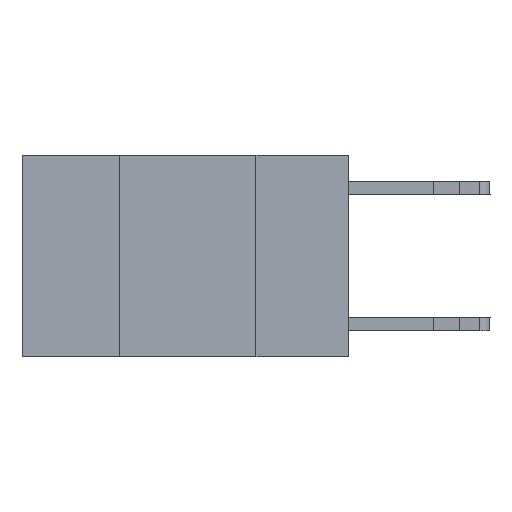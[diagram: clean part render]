
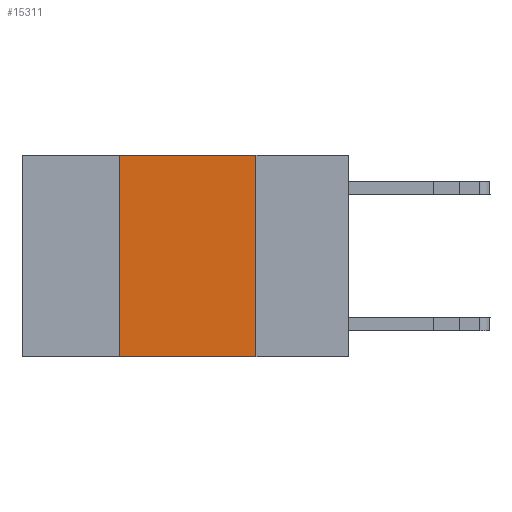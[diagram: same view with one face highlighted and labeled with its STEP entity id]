
A CAD part, left-side view. The second image highlights one B-rep face of the part: STEP entity #15311.
In plain terms, the highlighted planar face has unit normal (-1, 0, 0).
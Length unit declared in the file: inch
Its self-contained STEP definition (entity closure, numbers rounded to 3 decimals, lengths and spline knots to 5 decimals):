
#153 = PLANE ( 'NONE',  #7304 ) ;
#226 = DIRECTION ( 'NONE',  ( 0., -1., 0. ) ) ;
#289 = VERTEX_POINT ( 'NONE', #11946 ) ;
#1091 = EDGE_CURVE ( 'NONE', #289, #7516, #4039, .T. ) ;
#1394 = CARTESIAN_POINT ( 'NONE',  ( 0., 0.6, 0. ) ) ;
#1438 = VERTEX_POINT ( 'NONE', #4000 ) ;
#1507 = CARTESIAN_POINT ( 'NONE',  ( 0., 0.6, -0.37 ) ) ;
#2145 = EDGE_CURVE ( 'NONE', #1438, #4089, #7853, .T. ) ;
#2766 = ORIENTED_EDGE ( 'NONE', *, *, #5852, .F. ) ;
#3180 = VECTOR ( 'NONE', #7552, 39.37008 ) ;
#3196 = EDGE_CURVE ( 'NONE', #1438, #289, #8893, .T. ) ;
#3746 = DIRECTION ( 'NONE',  ( 0., 0., -1. ) ) ;
#4000 = CARTESIAN_POINT ( 'NONE',  ( 0., 0.42, -0.37 ) ) ;
#4039 = LINE ( 'NONE', #1394, #7570 ) ;
#4089 = VERTEX_POINT ( 'NONE', #15460 ) ;
#4158 = ORIENTED_EDGE ( 'NONE', *, *, #1091, .F. ) ;
#4558 = EDGE_LOOP ( 'NONE', ( #2766, #4158, #15081, #15997 ) ) ;
#4674 = DIRECTION ( 'NONE',  ( 0., 0., -1. ) ) ;
#4994 = LINE ( 'NONE', #15204, #8172 ) ;
#5852 = EDGE_CURVE ( 'NONE', #7516, #4089, #4994, .T. ) ;
#5996 = CARTESIAN_POINT ( 'NONE',  ( 0., 0.17, 0. ) ) ;
#6511 = CARTESIAN_POINT ( 'NONE',  ( 0., 0.6, 0. ) ) ;
#7304 = AXIS2_PLACEMENT_3D ( 'NONE', #6511, #15384, #4674 ) ;
#7516 = VERTEX_POINT ( 'NONE', #5996 ) ;
#7552 = DIRECTION ( 'NONE',  ( 0., 0., 1. ) ) ;
#7570 = VECTOR ( 'NONE', #11741, 39.37008 ) ;
#7853 = LINE ( 'NONE', #1507, #9814 ) ;
#8172 = VECTOR ( 'NONE', #3746, 39.37008 ) ;
#8893 = LINE ( 'NONE', #13975, #3180 ) ;
#9814 = VECTOR ( 'NONE', #226, 39.37008 ) ;
#11741 = DIRECTION ( 'NONE',  ( 0., -1., 0. ) ) ;
#11946 = CARTESIAN_POINT ( 'NONE',  ( 0., 0.42, 0. ) ) ;
#13975 = CARTESIAN_POINT ( 'NONE',  ( 0., 0.42, 0. ) ) ;
#15081 = ORIENTED_EDGE ( 'NONE', *, *, #3196, .F. ) ;
#15135 = FACE_OUTER_BOUND ( 'NONE', #4558, .T. ) ;
#15204 = CARTESIAN_POINT ( 'NONE',  ( 0., 0.17, 0. ) ) ;
#15311 = ADVANCED_FACE ( 'NONE', ( #15135 ), #153, .F. ) ;
#15384 = DIRECTION ( 'NONE',  ( 1., 0., 0. ) ) ;
#15460 = CARTESIAN_POINT ( 'NONE',  ( 0., 0.17, -0.37 ) ) ;
#15997 = ORIENTED_EDGE ( 'NONE', *, *, #2145, .T. ) ;
